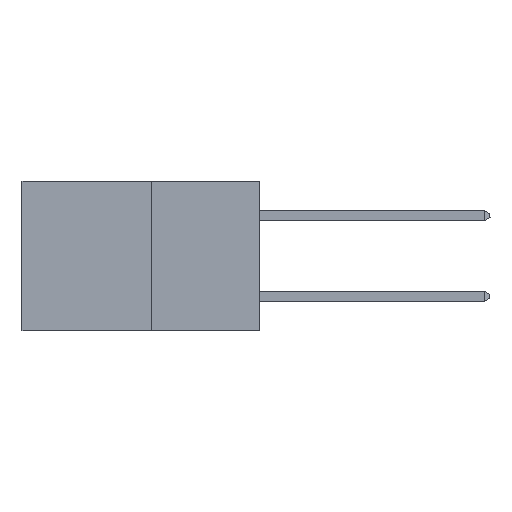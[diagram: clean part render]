
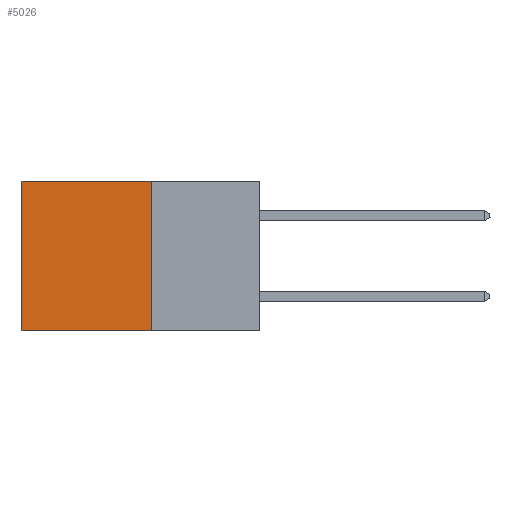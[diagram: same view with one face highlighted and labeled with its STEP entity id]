
A CAD part, left-side view. The second image highlights one B-rep face of the part: STEP entity #5026.
In plain terms, the highlighted planar face has unit normal (-1, 0, 0).
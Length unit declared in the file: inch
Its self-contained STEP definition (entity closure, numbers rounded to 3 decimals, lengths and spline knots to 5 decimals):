
#454 = DIRECTION ( 'NONE',  ( 0., 1., 0. ) ) ;
#1109 = DIRECTION ( 'NONE',  ( 1., 0., 0. ) ) ;
#1718 = CARTESIAN_POINT ( 'NONE',  ( 0.277, 0.27, 0. ) ) ;
#1740 = CARTESIAN_POINT ( 'NONE',  ( 0.277, 0.59, 0. ) ) ;
#2412 = CARTESIAN_POINT ( 'NONE',  ( 0.277, 0.59, -0.37 ) ) ;
#2741 = LINE ( 'NONE', #1718, #6051 ) ;
#2979 = VECTOR ( 'NONE', #454, 39.37008 ) ;
#3647 = ORIENTED_EDGE ( 'NONE', *, *, #12189, .F. ) ;
#3852 = DIRECTION ( 'NONE',  ( 0., 0., -1. ) ) ;
#5026 = ADVANCED_FACE ( 'NONE', ( #15374 ), #5280, .F. ) ;
#5280 = PLANE ( 'NONE',  #11535 ) ;
#5322 = CARTESIAN_POINT ( 'NONE',  ( 0.277, 0.27, -0.37 ) ) ;
#5373 = VECTOR ( 'NONE', #3852, 39.37008 ) ;
#6051 = VECTOR ( 'NONE', #12865, 39.37008 ) ;
#6160 = CARTESIAN_POINT ( 'NONE',  ( 0.277, 0.27, -0.37 ) ) ;
#6267 = EDGE_LOOP ( 'NONE', ( #11691, #3647, #15017, #17460 ) ) ;
#6466 = CARTESIAN_POINT ( 'NONE',  ( 0.277, 0.59, -0.37 ) ) ;
#6713 = EDGE_CURVE ( 'NONE', #11215, #12145, #2741, .T. ) ;
#6731 = LINE ( 'NONE', #11558, #2979 ) ;
#6861 = CARTESIAN_POINT ( 'NONE',  ( 0.277, 0.27, 0. ) ) ;
#9297 = VECTOR ( 'NONE', #13492, 39.37008 ) ;
#10870 = DIRECTION ( 'NONE',  ( 0., 0., -1. ) ) ;
#11215 = VERTEX_POINT ( 'NONE', #6861 ) ;
#11535 = AXIS2_PLACEMENT_3D ( 'NONE', #16276, #1109, #10870 ) ;
#11558 = CARTESIAN_POINT ( 'NONE',  ( 0.277, 0.27, -0.37 ) ) ;
#11691 = ORIENTED_EDGE ( 'NONE', *, *, #16018, .T. ) ;
#12145 = VERTEX_POINT ( 'NONE', #1740 ) ;
#12189 = EDGE_CURVE ( 'NONE', #15847, #16667, #6731, .T. ) ;
#12308 = LINE ( 'NONE', #5322, #5373 ) ;
#12865 = DIRECTION ( 'NONE',  ( 0., 1., 0. ) ) ;
#13492 = DIRECTION ( 'NONE',  ( 0., 0., -1. ) ) ;
#15017 = ORIENTED_EDGE ( 'NONE', *, *, #16697, .F. ) ;
#15374 = FACE_OUTER_BOUND ( 'NONE', #6267, .T. ) ;
#15847 = VERTEX_POINT ( 'NONE', #6160 ) ;
#16018 = EDGE_CURVE ( 'NONE', #12145, #16667, #16984, .T. ) ;
#16276 = CARTESIAN_POINT ( 'NONE',  ( 0.277, 0.27, -0.37 ) ) ;
#16667 = VERTEX_POINT ( 'NONE', #2412 ) ;
#16697 = EDGE_CURVE ( 'NONE', #11215, #15847, #12308, .T. ) ;
#16984 = LINE ( 'NONE', #6466, #9297 ) ;
#17460 = ORIENTED_EDGE ( 'NONE', *, *, #6713, .T. ) ;
